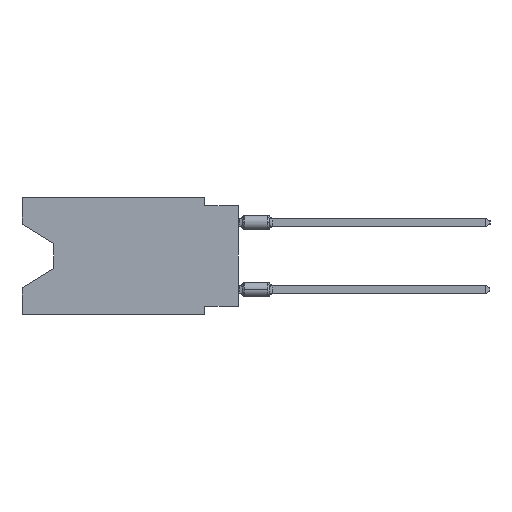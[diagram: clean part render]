
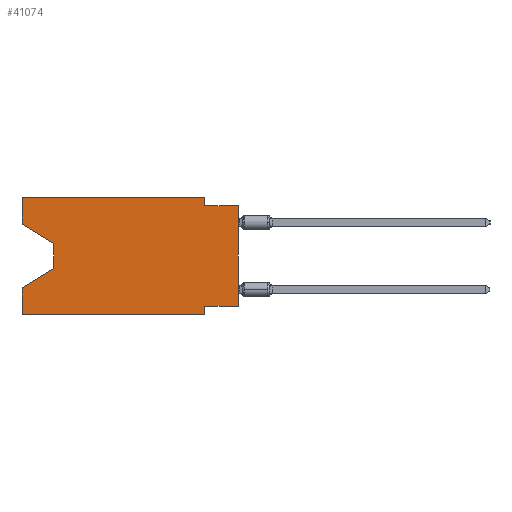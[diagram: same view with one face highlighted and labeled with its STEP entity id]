
A CAD part, left-side view. The second image highlights one B-rep face of the part: STEP entity #41074.
In plain terms, the highlighted planar face has unit normal (-1, 0, 0).
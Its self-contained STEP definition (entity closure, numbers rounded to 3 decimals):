
#1380 = CARTESIAN_POINT ( 'NONE',  ( 0., 0., -8.255 ) ) ;
#2173 = LINE ( 'NONE', #10519, #9881 ) ;
#2567 = ORIENTED_EDGE ( 'NONE', *, *, #55163, .T. ) ;
#2666 = VERTEX_POINT ( 'NONE', #21191 ) ;
#2723 = VERTEX_POINT ( 'NONE', #13030 ) ;
#3377 = LINE ( 'NONE', #28967, #21947 ) ;
#3546 = EDGE_CURVE ( 'NONE', #2666, #11253, #38985, .T. ) ;
#3583 = FACE_OUTER_BOUND ( 'NONE', #44086, .T. ) ;
#3901 = EDGE_CURVE ( 'NONE', #24292, #11253, #4694, .T. ) ;
#4031 = VECTOR ( 'NONE', #34386, 1000. ) ;
#4694 = LINE ( 'NONE', #13040, #43965 ) ;
#4716 = VECTOR ( 'NONE', #38493, 1000. ) ;
#4903 = LINE ( 'NONE', #5202, #31380 ) ;
#5202 = CARTESIAN_POINT ( 'NONE',  ( 0., 16.383, -8.89 ) ) ;
#6266 = CARTESIAN_POINT ( 'NONE',  ( 0., 2.54, -8.89 ) ) ;
#6704 = EDGE_CURVE ( 'NONE', #20326, #45699, #3377, .T. ) ;
#7242 = VECTOR ( 'NONE', #35232, 1000. ) ;
#7269 = EDGE_CURVE ( 'NONE', #41455, #52289, #34894, .T. ) ;
#7550 = LINE ( 'NONE', #46055, #19896 ) ;
#7921 = ORIENTED_EDGE ( 'NONE', *, *, #6704, .T. ) ;
#8758 = EDGE_CURVE ( 'NONE', #45384, #2666, #7550, .T. ) ;
#9305 = VECTOR ( 'NONE', #43701, 1000. ) ;
#9881 = VECTOR ( 'NONE', #31802, 1000. ) ;
#10084 = VERTEX_POINT ( 'NONE', #20221 ) ;
#10519 = CARTESIAN_POINT ( 'NONE',  ( 0., 0., -0.635 ) ) ;
#11091 = LINE ( 'NONE', #37243, #47070 ) ;
#11253 = VERTEX_POINT ( 'NONE', #14796 ) ;
#12121 = CARTESIAN_POINT ( 'NONE',  ( 0., 16.383, 0. ) ) ;
#12327 = CARTESIAN_POINT ( 'NONE',  ( 0., 13.97, -3.505 ) ) ;
#13030 = CARTESIAN_POINT ( 'NONE',  ( 0., 16.383, 0. ) ) ;
#13040 = CARTESIAN_POINT ( 'NONE',  ( 0., 16.383, 0. ) ) ;
#14796 = CARTESIAN_POINT ( 'NONE',  ( 0., 16.383, -6.852 ) ) ;
#14921 = ORIENTED_EDGE ( 'NONE', *, *, #35811, .T. ) ;
#16647 = CARTESIAN_POINT ( 'NONE',  ( 0., 2.54, -8.89 ) ) ;
#16796 = PLANE ( 'NONE',  #49579 ) ;
#18861 = DIRECTION ( 'NONE',  ( 0., 1., 0. ) ) ;
#19655 = EDGE_CURVE ( 'NONE', #2723, #41455, #30216, .T. ) ;
#19896 = VECTOR ( 'NONE', #24529, 1000. ) ;
#20002 = EDGE_CURVE ( 'NONE', #55313, #43385, #56023, .T. ) ;
#20221 = CARTESIAN_POINT ( 'NONE',  ( 0., 16.383, -2.038 ) ) ;
#20326 = VERTEX_POINT ( 'NONE', #1380 ) ;
#21191 = CARTESIAN_POINT ( 'NONE',  ( 0., 13.97, -5.385 ) ) ;
#21565 = ORIENTED_EDGE ( 'NONE', *, *, #39713, .F. ) ;
#21947 = VECTOR ( 'NONE', #55975, 1000. ) ;
#23285 = CARTESIAN_POINT ( 'NONE',  ( 0., 2.54, 0. ) ) ;
#24292 = VERTEX_POINT ( 'NONE', #24412 ) ;
#24412 = CARTESIAN_POINT ( 'NONE',  ( 0., 16.383, -8.89 ) ) ;
#24529 = DIRECTION ( 'NONE',  ( 0., 0., -1. ) ) ;
#25755 = CARTESIAN_POINT ( 'NONE',  ( 0., 16.383, -2.038 ) ) ;
#26635 = ORIENTED_EDGE ( 'NONE', *, *, #20002, .F. ) ;
#26770 = EDGE_CURVE ( 'NONE', #10084, #2723, #41542, .T. ) ;
#26815 = DIRECTION ( 'NONE',  ( 0., 0., -1. ) ) ;
#26839 = ORIENTED_EDGE ( 'NONE', *, *, #19655, .F. ) ;
#27506 = DIRECTION ( 'NONE',  ( 0., 0., 1. ) ) ;
#27614 = VECTOR ( 'NONE', #48094, 1000. ) ;
#28967 = CARTESIAN_POINT ( 'NONE',  ( 0., 0., 0. ) ) ;
#30216 = LINE ( 'NONE', #12121, #9305 ) ;
#30568 = CARTESIAN_POINT ( 'NONE',  ( 0., 2.54, 0. ) ) ;
#30988 = VECTOR ( 'NONE', #27506, 1000. ) ;
#31380 = VECTOR ( 'NONE', #35384, 1000. ) ;
#31643 = CARTESIAN_POINT ( 'NONE',  ( 0., 2.54, -8.255 ) ) ;
#31802 = DIRECTION ( 'NONE',  ( 0., -1., 0. ) ) ;
#32265 = DIRECTION ( 'NONE',  ( 1., 0., 0. ) ) ;
#32425 = EDGE_CURVE ( 'NONE', #20326, #55313, #11091, .T. ) ;
#33458 = ORIENTED_EDGE ( 'NONE', *, *, #3901, .F. ) ;
#34345 = DIRECTION ( 'NONE',  ( 0., 0., 1. ) ) ;
#34386 = DIRECTION ( 'NONE',  ( 0., -0.855, -0.519 ) ) ;
#34894 = LINE ( 'NONE', #30568, #27614 ) ;
#35232 = DIRECTION ( 'NONE',  ( 0., 0.855, -0.519 ) ) ;
#35384 = DIRECTION ( 'NONE',  ( 0., -1., 0. ) ) ;
#35811 = EDGE_CURVE ( 'NONE', #10084, #45384, #48133, .T. ) ;
#36407 = CARTESIAN_POINT ( 'NONE',  ( 0., 16.383, 0. ) ) ;
#36482 = ORIENTED_EDGE ( 'NONE', *, *, #7269, .F. ) ;
#37243 = CARTESIAN_POINT ( 'NONE',  ( 0., 0., -8.255 ) ) ;
#37714 = ORIENTED_EDGE ( 'NONE', *, *, #32425, .F. ) ;
#38136 = ORIENTED_EDGE ( 'NONE', *, *, #3546, .T. ) ;
#38493 = DIRECTION ( 'NONE',  ( 0., 0., -1. ) ) ;
#38985 = LINE ( 'NONE', #47330, #7242 ) ;
#39713 = EDGE_CURVE ( 'NONE', #52289, #45699, #2173, .T. ) ;
#41074 = ADVANCED_FACE ( 'NONE', ( #3583 ), #16796, .F. ) ;
#41455 = VERTEX_POINT ( 'NONE', #23285 ) ;
#41542 = LINE ( 'NONE', #36407, #30988 ) ;
#41658 = ORIENTED_EDGE ( 'NONE', *, *, #8758, .T. ) ;
#41873 = CARTESIAN_POINT ( 'NONE',  ( 0., 0., -0.635 ) ) ;
#43385 = VERTEX_POINT ( 'NONE', #6266 ) ;
#43701 = DIRECTION ( 'NONE',  ( 0., -1., 0. ) ) ;
#43965 = VECTOR ( 'NONE', #34345, 1000. ) ;
#44086 = EDGE_LOOP ( 'NONE', ( #14921, #41658, #38136, #33458, #2567, #26635, #37714, #7921, #21565, #36482, #26839, #46039 ) ) ;
#45384 = VERTEX_POINT ( 'NONE', #12327 ) ;
#45699 = VERTEX_POINT ( 'NONE', #41873 ) ;
#46039 = ORIENTED_EDGE ( 'NONE', *, *, #26770, .F. ) ;
#46055 = CARTESIAN_POINT ( 'NONE',  ( 0., 13.97, -3.505 ) ) ;
#47070 = VECTOR ( 'NONE', #18861, 1000. ) ;
#47330 = CARTESIAN_POINT ( 'NONE',  ( 0., 13.97, -5.385 ) ) ;
#48094 = DIRECTION ( 'NONE',  ( 0., 0., -1. ) ) ;
#48133 = LINE ( 'NONE', #25755, #4031 ) ;
#49579 = AXIS2_PLACEMENT_3D ( 'NONE', #52420, #32265, #26815 ) ;
#52289 = VERTEX_POINT ( 'NONE', #52690 ) ;
#52420 = CARTESIAN_POINT ( 'NONE',  ( 0., 16.383, 0. ) ) ;
#52690 = CARTESIAN_POINT ( 'NONE',  ( 0., 2.54, -0.635 ) ) ;
#55163 = EDGE_CURVE ( 'NONE', #24292, #43385, #4903, .T. ) ;
#55313 = VERTEX_POINT ( 'NONE', #31643 ) ;
#55975 = DIRECTION ( 'NONE',  ( 0., 0., 1. ) ) ;
#56023 = LINE ( 'NONE', #16647, #4716 ) ;
